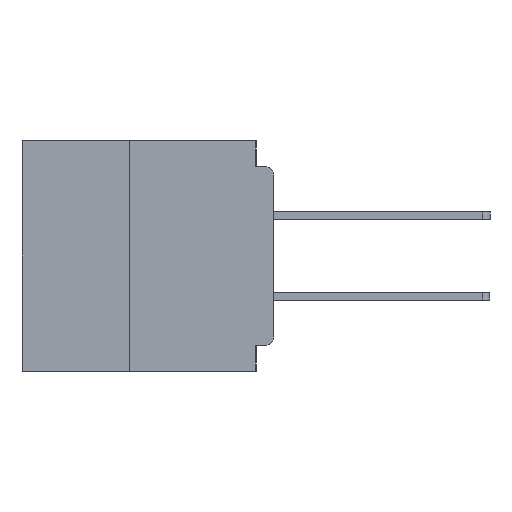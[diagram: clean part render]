
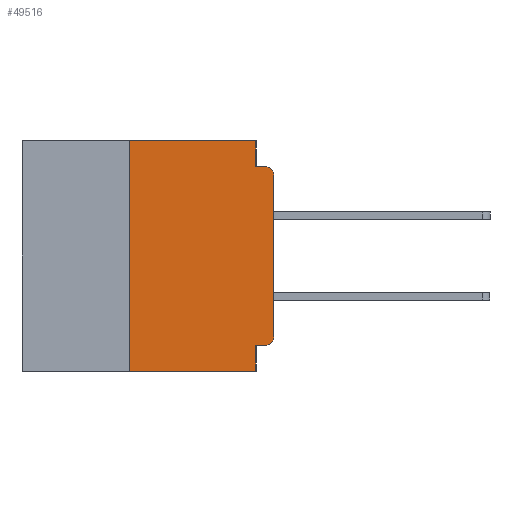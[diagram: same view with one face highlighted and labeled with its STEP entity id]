
A CAD part, left-side view. The second image highlights one B-rep face of the part: STEP entity #49516.
In plain terms, the highlighted planar face has unit normal (-1, 0, 0).
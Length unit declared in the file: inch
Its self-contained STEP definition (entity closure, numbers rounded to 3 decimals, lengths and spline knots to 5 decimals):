
#301 = CARTESIAN_POINT ( 'NONE',  ( 0., 0.031, 0. ) ) ;
#1325 = DIRECTION ( 'NONE',  ( 0., 0., -1. ) ) ;
#2926 = LINE ( 'NONE', #301, #20649 ) ;
#3242 = AXIS2_PLACEMENT_3D ( 'NONE', #34781, #10573, #38831 ) ;
#3247 = VECTOR ( 'NONE', #43330, 39.37008 ) ;
#4024 = ORIENTED_EDGE ( 'NONE', *, *, #34003, .F. ) ;
#4073 = LINE ( 'NONE', #8181, #24345 ) ;
#4636 = ORIENTED_EDGE ( 'NONE', *, *, #38410, .F. ) ;
#7839 = ORIENTED_EDGE ( 'NONE', *, *, #31776, .T. ) ;
#8181 = CARTESIAN_POINT ( 'NONE',  ( 0., 0.437, 0. ) ) ;
#8449 = ORIENTED_EDGE ( 'NONE', *, *, #35728, .F. ) ;
#8514 = DIRECTION ( 'NONE',  ( 0., -1., 0. ) ) ;
#9500 = CARTESIAN_POINT ( 'NONE',  ( 0., 0., 0. ) ) ;
#9509 = CARTESIAN_POINT ( 'NONE',  ( 0., 0.25, -0.4 ) ) ;
#10032 = AXIS2_PLACEMENT_3D ( 'NONE', #20049, #48264, #24107 ) ;
#10395 = LINE ( 'NONE', #49685, #30633 ) ;
#10513 = CARTESIAN_POINT ( 'NONE',  ( 0., 0.015, -0.045 ) ) ;
#10573 = DIRECTION ( 'NONE',  ( 1., 0., 0. ) ) ;
#11277 = DIRECTION ( 'NONE',  ( 0., 0., -1. ) ) ;
#11285 = VERTEX_POINT ( 'NONE', #44961 ) ;
#11789 = EDGE_CURVE ( 'NONE', #32433, #44283, #41885, .T. ) ;
#12265 = DIRECTION ( 'NONE',  ( 0., -1., 0. ) ) ;
#13441 = DIRECTION ( 'NONE',  ( 0., 0., 1. ) ) ;
#14012 = LINE ( 'NONE', #51227, #3247 ) ;
#14536 = CARTESIAN_POINT ( 'NONE',  ( 0., 0.015, -0.34 ) ) ;
#14614 = VERTEX_POINT ( 'NONE', #9509 ) ;
#16238 = EDGE_CURVE ( 'NONE', #19296, #26244, #36156, .T. ) ;
#16572 = DIRECTION ( 'NONE',  ( 0., -1., 0. ) ) ;
#18613 = DIRECTION ( 'NONE',  ( 0., 0., -1. ) ) ;
#19296 = VERTEX_POINT ( 'NONE', #23269 ) ;
#19494 = EDGE_CURVE ( 'NONE', #14614, #21603, #31094, .T. ) ;
#20049 = CARTESIAN_POINT ( 'NONE',  ( 0., 0.015, -0.06 ) ) ;
#20347 = VECTOR ( 'NONE', #16572, 39.37008 ) ;
#20649 = VECTOR ( 'NONE', #11277, 39.37008 ) ;
#21603 = VERTEX_POINT ( 'NONE', #49816 ) ;
#21965 = CIRCLE ( 'NONE', #25331, 0.015 ) ;
#22004 = VERTEX_POINT ( 'NONE', #28833 ) ;
#22368 = ORIENTED_EDGE ( 'NONE', *, *, #11789, .T. ) ;
#22597 = PLANE ( 'NONE',  #3242 ) ;
#23269 = CARTESIAN_POINT ( 'NONE',  ( 0., 0.015, -0.355 ) ) ;
#23703 = VECTOR ( 'NONE', #13441, 39.37008 ) ;
#24107 = DIRECTION ( 'NONE',  ( 0., 0., -1. ) ) ;
#24159 = VECTOR ( 'NONE', #43940, 39.37008 ) ;
#24345 = VECTOR ( 'NONE', #12265, 39.37008 ) ;
#24926 = ORIENTED_EDGE ( 'NONE', *, *, #31470, .F. ) ;
#25139 = CARTESIAN_POINT ( 'NONE',  ( 0., 0.031, 0. ) ) ;
#25331 = AXIS2_PLACEMENT_3D ( 'NONE', #14536, #42755, #18613 ) ;
#26244 = VERTEX_POINT ( 'NONE', #47704 ) ;
#26411 = LINE ( 'NONE', #28489, #35894 ) ;
#26836 = FACE_OUTER_BOUND ( 'NONE', #30348, .T. ) ;
#28489 = CARTESIAN_POINT ( 'NONE',  ( 0., 0., -0.045 ) ) ;
#28833 = CARTESIAN_POINT ( 'NONE',  ( 0., 0.25, 0. ) ) ;
#30348 = EDGE_LOOP ( 'NONE', ( #42572, #22368, #24926, #4636, #36886, #8449, #40688, #4024, #38817, #7839 ) ) ;
#30633 = VECTOR ( 'NONE', #1325, 39.37008 ) ;
#31094 = LINE ( 'NONE', #48821, #20347 ) ;
#31470 = EDGE_CURVE ( 'NONE', #51395, #44283, #26411, .T. ) ;
#31776 = EDGE_CURVE ( 'NONE', #19296, #11285, #21965, .T. ) ;
#32433 = VERTEX_POINT ( 'NONE', #47627 ) ;
#34003 = EDGE_CURVE ( 'NONE', #26244, #21603, #10395, .T. ) ;
#34379 = CARTESIAN_POINT ( 'NONE',  ( 0., 0.031, -0.045 ) ) ;
#34781 = CARTESIAN_POINT ( 'NONE',  ( 0., 0.437, 0. ) ) ;
#35728 = EDGE_CURVE ( 'NONE', #14614, #22004, #14012, .T. ) ;
#35894 = VECTOR ( 'NONE', #8514, 39.37008 ) ;
#36029 = VERTEX_POINT ( 'NONE', #25139 ) ;
#36156 = LINE ( 'NONE', #51836, #24159 ) ;
#36886 = ORIENTED_EDGE ( 'NONE', *, *, #39212, .F. ) ;
#38410 = EDGE_CURVE ( 'NONE', #36029, #51395, #2926, .T. ) ;
#38817 = ORIENTED_EDGE ( 'NONE', *, *, #16238, .F. ) ;
#38831 = DIRECTION ( 'NONE',  ( 0., 0., -1. ) ) ;
#39212 = EDGE_CURVE ( 'NONE', #22004, #36029, #4073, .T. ) ;
#40688 = ORIENTED_EDGE ( 'NONE', *, *, #19494, .T. ) ;
#41885 = CIRCLE ( 'NONE', #10032, 0.015 ) ;
#42572 = ORIENTED_EDGE ( 'NONE', *, *, #49348, .T. ) ;
#42755 = DIRECTION ( 'NONE',  ( -1., 0., 0. ) ) ;
#43330 = DIRECTION ( 'NONE',  ( 0., 0., 1. ) ) ;
#43940 = DIRECTION ( 'NONE',  ( 0., 1., 0. ) ) ;
#44283 = VERTEX_POINT ( 'NONE', #10513 ) ;
#44961 = CARTESIAN_POINT ( 'NONE',  ( 0., 0., -0.34 ) ) ;
#45154 = LINE ( 'NONE', #9500, #23703 ) ;
#47627 = CARTESIAN_POINT ( 'NONE',  ( 0., 0., -0.06 ) ) ;
#47704 = CARTESIAN_POINT ( 'NONE',  ( 0., 0.031, -0.355 ) ) ;
#48264 = DIRECTION ( 'NONE',  ( -1., 0., 0. ) ) ;
#48821 = CARTESIAN_POINT ( 'NONE',  ( 0., 0.437, -0.4 ) ) ;
#49348 = EDGE_CURVE ( 'NONE', #11285, #32433, #45154, .T. ) ;
#49516 = ADVANCED_FACE ( 'NONE', ( #26836 ), #22597, .F. ) ;
#49685 = CARTESIAN_POINT ( 'NONE',  ( 0., 0.031, -0.4 ) ) ;
#49816 = CARTESIAN_POINT ( 'NONE',  ( 0., 0.031, -0.4 ) ) ;
#51227 = CARTESIAN_POINT ( 'NONE',  ( 0., 0.25, -0.4 ) ) ;
#51395 = VERTEX_POINT ( 'NONE', #34379 ) ;
#51836 = CARTESIAN_POINT ( 'NONE',  ( 0., 0., -0.355 ) ) ;
